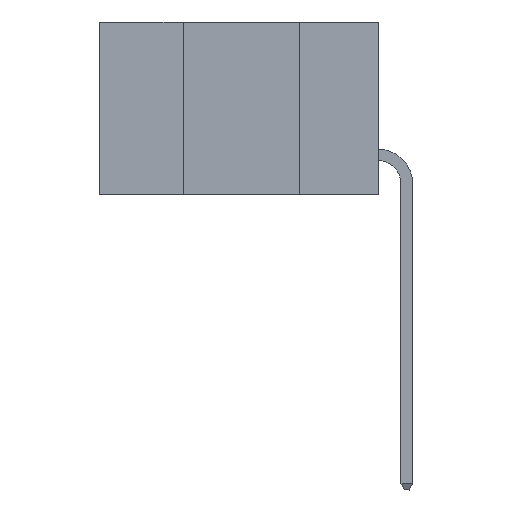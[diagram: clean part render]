
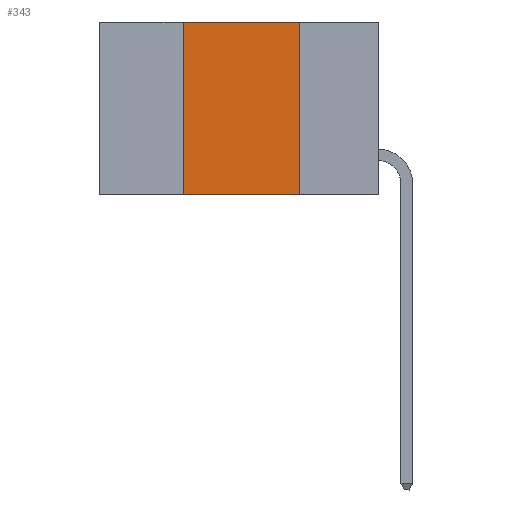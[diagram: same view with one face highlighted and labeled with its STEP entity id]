
A CAD part, left-side view. The second image highlights one B-rep face of the part: STEP entity #343.
In plain terms, the highlighted planar face has unit normal (-1, 0, 0).
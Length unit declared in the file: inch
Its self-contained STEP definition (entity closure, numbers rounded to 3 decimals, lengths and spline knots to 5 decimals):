
#225 = DIRECTION ( 'NONE',  ( 0., -1., 0. ) ) ;
#228 = LINE ( 'NONE', #3040, #323 ) ;
#323 = VECTOR ( 'NONE', #7384, 39.37008 ) ;
#343 = ADVANCED_FACE ( 'NONE', ( #456 ), #4044, .F. ) ;
#456 = FACE_OUTER_BOUND ( 'NONE', #8852, .T. ) ;
#1146 = CARTESIAN_POINT ( 'NONE',  ( 0., 0.6, -0.37 ) ) ;
#1199 = VERTEX_POINT ( 'NONE', #6949 ) ;
#1355 = CARTESIAN_POINT ( 'NONE',  ( 0., 0.6, 0. ) ) ;
#1444 = DIRECTION ( 'NONE',  ( 0., 0., -1. ) ) ;
#1601 = VECTOR ( 'NONE', #10892, 39.37008 ) ;
#3040 = CARTESIAN_POINT ( 'NONE',  ( 0., 0.17, -0.37 ) ) ;
#3060 = ORIENTED_EDGE ( 'NONE', *, *, #10559, .F. ) ;
#3142 = CARTESIAN_POINT ( 'NONE',  ( 0., 0.6, 0. ) ) ;
#3288 = LINE ( 'NONE', #1355, #3594 ) ;
#3594 = VECTOR ( 'NONE', #9569, 39.37008 ) ;
#3761 = EDGE_CURVE ( 'NONE', #6316, #1199, #3288, .T. ) ;
#3950 = AXIS2_PLACEMENT_3D ( 'NONE', #3142, #7842, #1444 ) ;
#4044 = PLANE ( 'NONE',  #3950 ) ;
#4197 = ORIENTED_EDGE ( 'NONE', *, *, #11355, .T. ) ;
#4621 = VECTOR ( 'NONE', #225, 39.37008 ) ;
#4804 = VERTEX_POINT ( 'NONE', #7244 ) ;
#5411 = EDGE_CURVE ( 'NONE', #1199, #8248, #228, .T. ) ;
#6316 = VERTEX_POINT ( 'NONE', #8618 ) ;
#6941 = ORIENTED_EDGE ( 'NONE', *, *, #5411, .F. ) ;
#6949 = CARTESIAN_POINT ( 'NONE',  ( 0., 0.17, 0. ) ) ;
#6974 = CARTESIAN_POINT ( 'NONE',  ( 0., 0.17, -0.37 ) ) ;
#7244 = CARTESIAN_POINT ( 'NONE',  ( 0., 0.42, -0.37 ) ) ;
#7384 = DIRECTION ( 'NONE',  ( 0., 0., -1. ) ) ;
#7770 = CARTESIAN_POINT ( 'NONE',  ( 0., 0.42, -0.37 ) ) ;
#7842 = DIRECTION ( 'NONE',  ( 1., 0., 0. ) ) ;
#8248 = VERTEX_POINT ( 'NONE', #6974 ) ;
#8618 = CARTESIAN_POINT ( 'NONE',  ( 0., 0.42, 0. ) ) ;
#8852 = EDGE_LOOP ( 'NONE', ( #6941, #10646, #3060, #4197 ) ) ;
#9556 = LINE ( 'NONE', #1146, #4621 ) ;
#9569 = DIRECTION ( 'NONE',  ( 0., -1., 0. ) ) ;
#9587 = LINE ( 'NONE', #7770, #1601 ) ;
#10559 = EDGE_CURVE ( 'NONE', #4804, #6316, #9587, .T. ) ;
#10646 = ORIENTED_EDGE ( 'NONE', *, *, #3761, .F. ) ;
#10892 = DIRECTION ( 'NONE',  ( 0., 0., 1. ) ) ;
#11355 = EDGE_CURVE ( 'NONE', #4804, #8248, #9556, .T. ) ;
